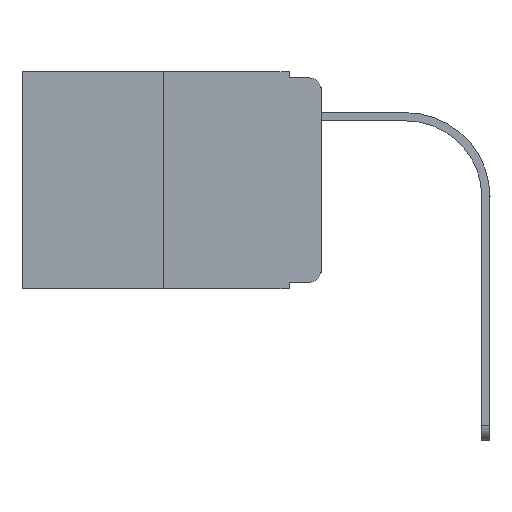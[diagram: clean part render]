
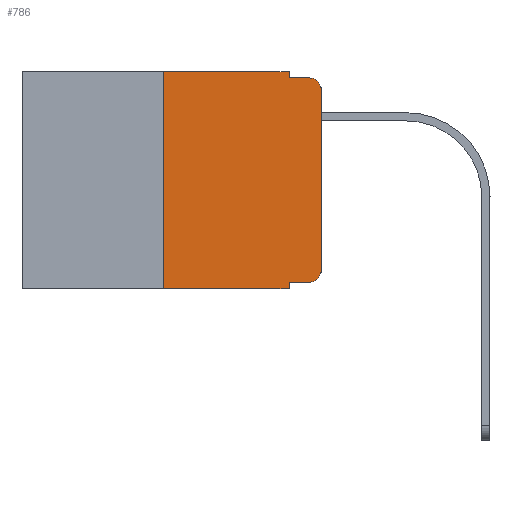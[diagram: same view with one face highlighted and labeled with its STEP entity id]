
A CAD part, left-side view. The second image highlights one B-rep face of the part: STEP entity #786.
In plain terms, the highlighted planar face has unit normal (-1, 0, 0).
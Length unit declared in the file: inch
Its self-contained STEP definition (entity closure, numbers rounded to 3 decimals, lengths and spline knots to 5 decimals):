
#20 = DIRECTION ( 'NONE',  ( 0., -1., 0. ) ) ;
#107 = VERTEX_POINT ( 'NONE', #9452 ) ;
#229 = FACE_OUTER_BOUND ( 'NONE', #9684, .T. ) ;
#370 = ORIENTED_EDGE ( 'NONE', *, *, #5869, .T. ) ;
#658 = VECTOR ( 'NONE', #8816, 39.37008 ) ;
#698 = CIRCLE ( 'NONE', #2836, 0.02 ) ;
#770 = VERTEX_POINT ( 'NONE', #10481 ) ;
#786 = ADVANCED_FACE ( 'NONE', ( #229 ), #2140, .F. ) ;
#939 = ORIENTED_EDGE ( 'NONE', *, *, #9261, .T. ) ;
#949 = CARTESIAN_POINT ( 'NONE',  ( 0., 0., -0.03 ) ) ;
#1043 = DIRECTION ( 'NONE',  ( -1., 0., 0. ) ) ;
#1065 = DIRECTION ( 'NONE',  ( 0., 0., -1. ) ) ;
#1116 = LINE ( 'NONE', #9268, #3734 ) ;
#1305 = CARTESIAN_POINT ( 'NONE',  ( 0., 0.051, -0.333 ) ) ;
#1355 = CARTESIAN_POINT ( 'NONE',  ( 0., 0.02, -0.03 ) ) ;
#1467 = ORIENTED_EDGE ( 'NONE', *, *, #7161, .T. ) ;
#1803 = CARTESIAN_POINT ( 'NONE',  ( 0., 0.473, 0. ) ) ;
#1852 = CARTESIAN_POINT ( 'NONE',  ( 0., 0.02, -0.333 ) ) ;
#2035 = DIRECTION ( 'NONE',  ( 1., 0., 0. ) ) ;
#2075 = DIRECTION ( 'NONE',  ( 0., -1., 0. ) ) ;
#2140 = PLANE ( 'NONE',  #7037 ) ;
#2155 = EDGE_CURVE ( 'NONE', #3093, #9260, #698, .T. ) ;
#2623 = ORIENTED_EDGE ( 'NONE', *, *, #2155, .T. ) ;
#2719 = VECTOR ( 'NONE', #5043, 39.37008 ) ;
#2759 = CARTESIAN_POINT ( 'NONE',  ( 0., 0.051, 0. ) ) ;
#2761 = VECTOR ( 'NONE', #5445, 39.37008 ) ;
#2836 = AXIS2_PLACEMENT_3D ( 'NONE', #1355, #3245, #4027 ) ;
#2872 = CARTESIAN_POINT ( 'NONE',  ( 0., 0.02, -0.313 ) ) ;
#2899 = LINE ( 'NONE', #5679, #6284 ) ;
#2952 = LINE ( 'NONE', #1803, #7800 ) ;
#3093 = VERTEX_POINT ( 'NONE', #949 ) ;
#3245 = DIRECTION ( 'NONE',  ( -1., 0., 0. ) ) ;
#3321 = ORIENTED_EDGE ( 'NONE', *, *, #6834, .T. ) ;
#3594 = CARTESIAN_POINT ( 'NONE',  ( 0., 0.051, 0. ) ) ;
#3734 = VECTOR ( 'NONE', #4675, 39.37008 ) ;
#3909 = EDGE_CURVE ( 'NONE', #6626, #107, #10775, .T. ) ;
#4027 = DIRECTION ( 'NONE',  ( 0., 0., -1. ) ) ;
#4471 = VERTEX_POINT ( 'NONE', #4710 ) ;
#4620 = CARTESIAN_POINT ( 'NONE',  ( 0., 0., 0. ) ) ;
#4675 = DIRECTION ( 'NONE',  ( 0., 0., 1. ) ) ;
#4690 = AXIS2_PLACEMENT_3D ( 'NONE', #2872, #1043, #7518 ) ;
#4710 = CARTESIAN_POINT ( 'NONE',  ( 0., 0.25, -0.343 ) ) ;
#4896 = ORIENTED_EDGE ( 'NONE', *, *, #7136, .F. ) ;
#5043 = DIRECTION ( 'NONE',  ( 0., -1., 0. ) ) ;
#5445 = DIRECTION ( 'NONE',  ( 0., 0., -1. ) ) ;
#5526 = LINE ( 'NONE', #4620, #10496 ) ;
#5631 = VERTEX_POINT ( 'NONE', #6326 ) ;
#5679 = CARTESIAN_POINT ( 'NONE',  ( 0., 0.473, -0.343 ) ) ;
#5869 = EDGE_CURVE ( 'NONE', #11708, #3093, #5526, .T. ) ;
#6003 = EDGE_CURVE ( 'NONE', #107, #9260, #10524, .T. ) ;
#6284 = VECTOR ( 'NONE', #11219, 39.37008 ) ;
#6326 = CARTESIAN_POINT ( 'NONE',  ( 0., 0.25, 0. ) ) ;
#6587 = LINE ( 'NONE', #1305, #2719 ) ;
#6626 = VERTEX_POINT ( 'NONE', #2759 ) ;
#6640 = CARTESIAN_POINT ( 'NONE',  ( 0., 0.473, 0. ) ) ;
#6834 = EDGE_CURVE ( 'NONE', #8980, #10687, #6587, .T. ) ;
#6842 = CARTESIAN_POINT ( 'NONE',  ( 0., 0.051, -0.333 ) ) ;
#6956 = ORIENTED_EDGE ( 'NONE', *, *, #3909, .F. ) ;
#7037 = AXIS2_PLACEMENT_3D ( 'NONE', #6640, #2035, #1065 ) ;
#7077 = ORIENTED_EDGE ( 'NONE', *, *, #6003, .F. ) ;
#7136 = EDGE_CURVE ( 'NONE', #4471, #5631, #1116, .T. ) ;
#7161 = EDGE_CURVE ( 'NONE', #10687, #11708, #7585, .T. ) ;
#7518 = DIRECTION ( 'NONE',  ( 0., 0., -1. ) ) ;
#7585 = CIRCLE ( 'NONE', #4690, 0.02 ) ;
#7726 = LINE ( 'NONE', #8753, #658 ) ;
#7800 = VECTOR ( 'NONE', #20, 39.37008 ) ;
#8294 = DIRECTION ( 'NONE',  ( 0., 0., 1. ) ) ;
#8412 = VECTOR ( 'NONE', #2075, 39.37008 ) ;
#8753 = CARTESIAN_POINT ( 'NONE',  ( 0., 0.051, 0. ) ) ;
#8816 = DIRECTION ( 'NONE',  ( 0., 0., -1. ) ) ;
#8833 = ORIENTED_EDGE ( 'NONE', *, *, #9050, .F. ) ;
#8980 = VERTEX_POINT ( 'NONE', #6842 ) ;
#9050 = EDGE_CURVE ( 'NONE', #8980, #770, #7726, .T. ) ;
#9260 = VERTEX_POINT ( 'NONE', #10265 ) ;
#9261 = EDGE_CURVE ( 'NONE', #4471, #770, #2899, .T. ) ;
#9268 = CARTESIAN_POINT ( 'NONE',  ( 0., 0.25, 0. ) ) ;
#9271 = EDGE_CURVE ( 'NONE', #5631, #6626, #2952, .T. ) ;
#9452 = CARTESIAN_POINT ( 'NONE',  ( 0., 0.051, -0.01 ) ) ;
#9684 = EDGE_LOOP ( 'NONE', ( #370, #2623, #7077, #6956, #11440, #4896, #939, #8833, #3321, #1467 ) ) ;
#10265 = CARTESIAN_POINT ( 'NONE',  ( 0., 0.02, -0.01 ) ) ;
#10355 = CARTESIAN_POINT ( 'NONE',  ( 0., 0.051, -0.01 ) ) ;
#10481 = CARTESIAN_POINT ( 'NONE',  ( 0., 0.051, -0.343 ) ) ;
#10496 = VECTOR ( 'NONE', #8294, 39.37008 ) ;
#10524 = LINE ( 'NONE', #10355, #8412 ) ;
#10687 = VERTEX_POINT ( 'NONE', #1852 ) ;
#10775 = LINE ( 'NONE', #3594, #2761 ) ;
#11219 = DIRECTION ( 'NONE',  ( 0., -1., 0. ) ) ;
#11438 = CARTESIAN_POINT ( 'NONE',  ( 0., 0., -0.313 ) ) ;
#11440 = ORIENTED_EDGE ( 'NONE', *, *, #9271, .F. ) ;
#11708 = VERTEX_POINT ( 'NONE', #11438 ) ;
